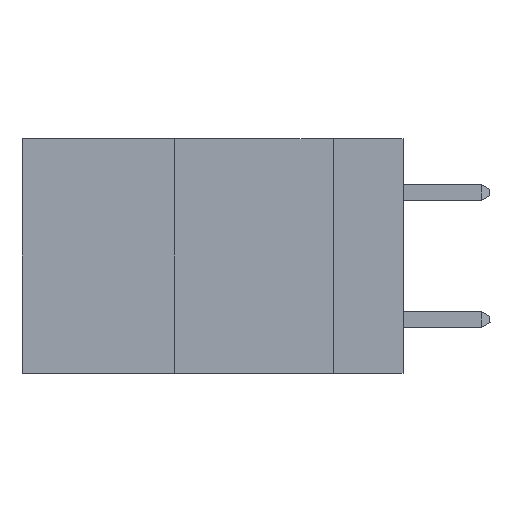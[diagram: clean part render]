
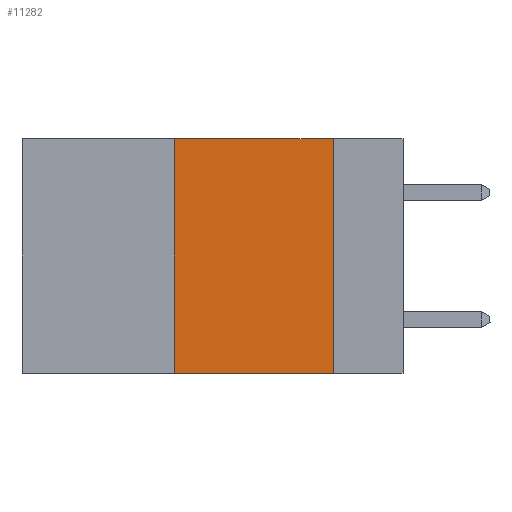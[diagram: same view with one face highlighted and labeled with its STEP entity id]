
A CAD part, left-side view. The second image highlights one B-rep face of the part: STEP entity #11282.
In plain terms, the highlighted planar face has unit normal (-1, 0, 0).
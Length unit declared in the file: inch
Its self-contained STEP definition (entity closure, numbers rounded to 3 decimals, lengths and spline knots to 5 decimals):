
#1179 = VECTOR ( 'NONE', #6893, 39.37008 ) ;
#1689 = PLANE ( 'NONE',  #2146 ) ;
#2146 = AXIS2_PLACEMENT_3D ( 'NONE', #10118, #12551, #14929 ) ;
#2238 = ORIENTED_EDGE ( 'NONE', *, *, #6193, .F. ) ;
#2284 = LINE ( 'NONE', #3181, #1179 ) ;
#2356 = DIRECTION ( 'NONE',  ( 0., 0., 1. ) ) ;
#2616 = VECTOR ( 'NONE', #7121, 39.37008 ) ;
#2753 = CARTESIAN_POINT ( 'NONE',  ( 0., 0.11, 0. ) ) ;
#2798 = DIRECTION ( 'NONE',  ( 0., -1., 0. ) ) ;
#2839 = LINE ( 'NONE', #5950, #8688 ) ;
#3181 = CARTESIAN_POINT ( 'NONE',  ( 0., 0.6, 0. ) ) ;
#3250 = CARTESIAN_POINT ( 'NONE',  ( 0., 0.11, 0. ) ) ;
#3794 = ORIENTED_EDGE ( 'NONE', *, *, #5600, .F. ) ;
#3849 = EDGE_LOOP ( 'NONE', ( #2238, #3794, #5043, #9652 ) ) ;
#5011 = EDGE_CURVE ( 'NONE', #12904, #6977, #6854, .T. ) ;
#5043 = ORIENTED_EDGE ( 'NONE', *, *, #5173, .F. ) ;
#5173 = EDGE_CURVE ( 'NONE', #12904, #5210, #2839, .T. ) ;
#5210 = VERTEX_POINT ( 'NONE', #8245 ) ;
#5600 = EDGE_CURVE ( 'NONE', #5210, #12183, #2284, .T. ) ;
#5950 = CARTESIAN_POINT ( 'NONE',  ( 0., 0.36, 0. ) ) ;
#6193 = EDGE_CURVE ( 'NONE', #12183, #6977, #6610, .T. ) ;
#6610 = LINE ( 'NONE', #3250, #2616 ) ;
#6854 = LINE ( 'NONE', #7459, #14936 ) ;
#6893 = DIRECTION ( 'NONE',  ( 0., -1., 0. ) ) ;
#6977 = VERTEX_POINT ( 'NONE', #13283 ) ;
#7121 = DIRECTION ( 'NONE',  ( 0., 0., -1. ) ) ;
#7459 = CARTESIAN_POINT ( 'NONE',  ( 0., 0.6, -0.37 ) ) ;
#8245 = CARTESIAN_POINT ( 'NONE',  ( 0., 0.36, 0. ) ) ;
#8688 = VECTOR ( 'NONE', #2356, 39.37008 ) ;
#8996 = CARTESIAN_POINT ( 'NONE',  ( 0., 0.36, -0.37 ) ) ;
#9652 = ORIENTED_EDGE ( 'NONE', *, *, #5011, .T. ) ;
#10118 = CARTESIAN_POINT ( 'NONE',  ( 0., 0.6, 0. ) ) ;
#11282 = ADVANCED_FACE ( 'NONE', ( #13452 ), #1689, .F. ) ;
#12183 = VERTEX_POINT ( 'NONE', #2753 ) ;
#12551 = DIRECTION ( 'NONE',  ( 1., 0., 0. ) ) ;
#12904 = VERTEX_POINT ( 'NONE', #8996 ) ;
#13283 = CARTESIAN_POINT ( 'NONE',  ( 0., 0.11, -0.37 ) ) ;
#13452 = FACE_OUTER_BOUND ( 'NONE', #3849, .T. ) ;
#14929 = DIRECTION ( 'NONE',  ( 0., 0., -1. ) ) ;
#14936 = VECTOR ( 'NONE', #2798, 39.37008 ) ;
